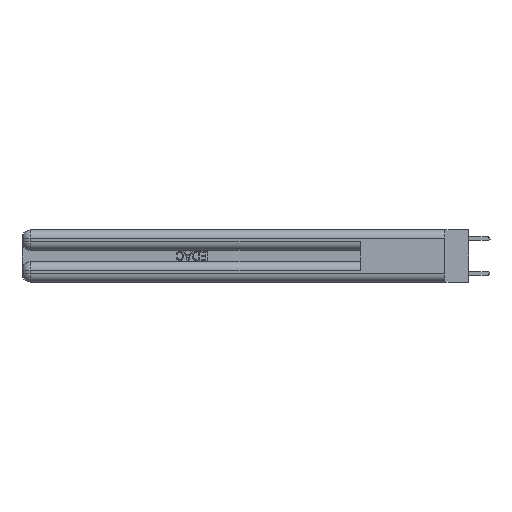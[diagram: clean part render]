
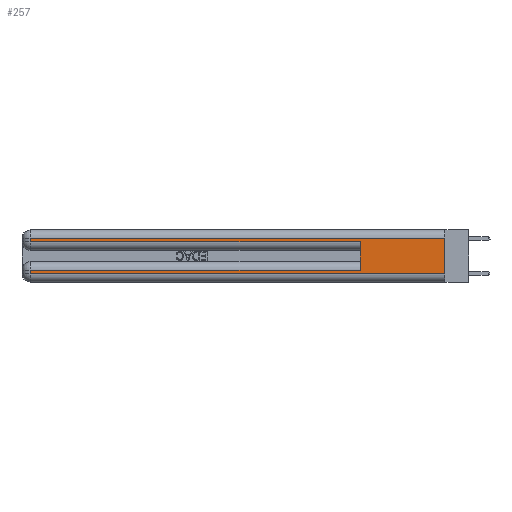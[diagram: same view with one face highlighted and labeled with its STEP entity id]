
A CAD part, left-side view. The second image highlights one B-rep face of the part: STEP entity #257.
In plain terms, the highlighted planar face has unit normal (-1, 0, 0).
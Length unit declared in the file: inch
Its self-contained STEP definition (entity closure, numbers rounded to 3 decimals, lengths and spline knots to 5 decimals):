
#188 = DIRECTION ( 'NONE',  ( 0., 1., 0. ) ) ;
#257 = ADVANCED_FACE ( 'NONE', ( #23014 ), #3483, .F. ) ;
#345 = EDGE_CURVE ( 'NONE', #31891, #6410, #21373, .T. ) ;
#668 = DIRECTION ( 'NONE',  ( 0., 0., -1. ) ) ;
#1401 = ORIENTED_EDGE ( 'NONE', *, *, #6431, .T. ) ;
#1917 = LINE ( 'NONE', #2355, #15046 ) ;
#2230 = VECTOR ( 'NONE', #5184, 39.37008 ) ;
#2355 = CARTESIAN_POINT ( 'NONE',  ( 0., 2.94, 0.37 ) ) ;
#3483 = PLANE ( 'NONE',  #24606 ) ;
#3613 = EDGE_CURVE ( 'NONE', #10356, #31205, #1917, .T. ) ;
#3652 = EDGE_CURVE ( 'NONE', #10367, #21644, #8079, .T. ) ;
#5018 = DIRECTION ( 'NONE',  ( 0., 0., -1. ) ) ;
#5184 = DIRECTION ( 'NONE',  ( 0., -1., 0. ) ) ;
#6120 = CARTESIAN_POINT ( 'NONE',  ( 0., 0., 0.37 ) ) ;
#6410 = VERTEX_POINT ( 'NONE', #15859 ) ;
#6431 = EDGE_CURVE ( 'NONE', #15477, #10356, #18198, .T. ) ;
#6464 = DIRECTION ( 'NONE',  ( 0., 1., 0. ) ) ;
#6643 = VECTOR ( 'NONE', #6464, 39.37008 ) ;
#6834 = VECTOR ( 'NONE', #668, 39.37008 ) ;
#7054 = ORIENTED_EDGE ( 'NONE', *, *, #3613, .T. ) ;
#7610 = ORIENTED_EDGE ( 'NONE', *, *, #19015, .T. ) ;
#8079 = LINE ( 'NONE', #18175, #21182 ) ;
#8763 = DIRECTION ( 'NONE',  ( 1., 0., 0. ) ) ;
#9229 = LINE ( 'NONE', #23501, #2230 ) ;
#10176 = EDGE_LOOP ( 'NONE', ( #33529, #20355, #25522, #13438, #31130, #1401, #7054, #7610 ) ) ;
#10241 = CARTESIAN_POINT ( 'NONE',  ( 0., 0.6, 0.145 ) ) ;
#10356 = VERTEX_POINT ( 'NONE', #29921 ) ;
#10367 = VERTEX_POINT ( 'NONE', #24695 ) ;
#10860 = CARTESIAN_POINT ( 'NONE',  ( 0., 2.94, 0.06 ) ) ;
#11023 = VECTOR ( 'NONE', #31125, 39.37008 ) ;
#12928 = DIRECTION ( 'NONE',  ( 0., -1., 0. ) ) ;
#13438 = ORIENTED_EDGE ( 'NONE', *, *, #3652, .T. ) ;
#15046 = VECTOR ( 'NONE', #5018, 39.37008 ) ;
#15477 = VERTEX_POINT ( 'NONE', #26827 ) ;
#15859 = CARTESIAN_POINT ( 'NONE',  ( 0., 2.94, 0.31 ) ) ;
#17316 = CARTESIAN_POINT ( 'NONE',  ( 0., 0.6, 0.285 ) ) ;
#18175 = CARTESIAN_POINT ( 'NONE',  ( 0., 0., 0.285 ) ) ;
#18198 = LINE ( 'NONE', #18515, #25142 ) ;
#18515 = CARTESIAN_POINT ( 'NONE',  ( 0., 0., 0.085 ) ) ;
#19015 = EDGE_CURVE ( 'NONE', #31205, #31309, #9229, .T. ) ;
#19114 = LINE ( 'NONE', #25722, #24417 ) ;
#20355 = ORIENTED_EDGE ( 'NONE', *, *, #345, .T. ) ;
#21182 = VECTOR ( 'NONE', #12928, 39.37008 ) ;
#21373 = LINE ( 'NONE', #27378, #6643 ) ;
#21644 = VERTEX_POINT ( 'NONE', #17316 ) ;
#23014 = FACE_OUTER_BOUND ( 'NONE', #10176, .T. ) ;
#23501 = CARTESIAN_POINT ( 'NONE',  ( 0., 0., 0.06 ) ) ;
#24134 = CARTESIAN_POINT ( 'NONE',  ( 0., 2.94, 0.37 ) ) ;
#24417 = VECTOR ( 'NONE', #28341, 39.37008 ) ;
#24606 = AXIS2_PLACEMENT_3D ( 'NONE', #6120, #8763, #27031 ) ;
#24695 = CARTESIAN_POINT ( 'NONE',  ( 0., 2.94, 0.285 ) ) ;
#25142 = VECTOR ( 'NONE', #188, 39.37008 ) ;
#25522 = ORIENTED_EDGE ( 'NONE', *, *, #26386, .T. ) ;
#25722 = CARTESIAN_POINT ( 'NONE',  ( 0., 0., 0.37 ) ) ;
#26136 = EDGE_CURVE ( 'NONE', #31891, #31309, #19114, .T. ) ;
#26386 = EDGE_CURVE ( 'NONE', #6410, #10367, #27691, .T. ) ;
#26827 = CARTESIAN_POINT ( 'NONE',  ( 0., 0.6, 0.085 ) ) ;
#27016 = CARTESIAN_POINT ( 'NONE',  ( 0., 0., 0.31 ) ) ;
#27031 = DIRECTION ( 'NONE',  ( 0., 0., -1. ) ) ;
#27378 = CARTESIAN_POINT ( 'NONE',  ( 0., 0., 0.31 ) ) ;
#27691 = LINE ( 'NONE', #24134, #6834 ) ;
#28341 = DIRECTION ( 'NONE',  ( 0., 0., -1. ) ) ;
#29921 = CARTESIAN_POINT ( 'NONE',  ( 0., 2.94, 0.085 ) ) ;
#31125 = DIRECTION ( 'NONE',  ( 0., 0., 1. ) ) ;
#31130 = ORIENTED_EDGE ( 'NONE', *, *, #31695, .F. ) ;
#31205 = VERTEX_POINT ( 'NONE', #10860 ) ;
#31309 = VERTEX_POINT ( 'NONE', #32049 ) ;
#31695 = EDGE_CURVE ( 'NONE', #15477, #21644, #31811, .T. ) ;
#31811 = LINE ( 'NONE', #10241, #11023 ) ;
#31891 = VERTEX_POINT ( 'NONE', #27016 ) ;
#32049 = CARTESIAN_POINT ( 'NONE',  ( 0., 0., 0.06 ) ) ;
#33529 = ORIENTED_EDGE ( 'NONE', *, *, #26136, .F. ) ;
